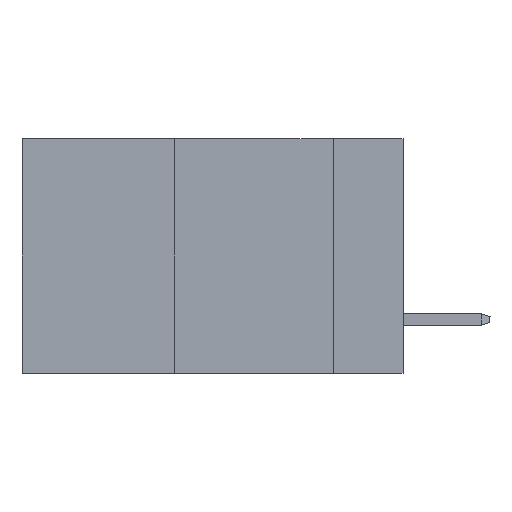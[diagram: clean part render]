
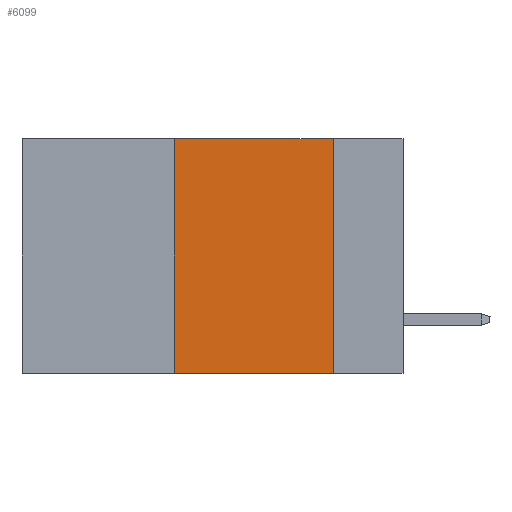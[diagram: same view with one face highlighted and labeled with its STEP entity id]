
A CAD part, left-side view. The second image highlights one B-rep face of the part: STEP entity #6099.
In plain terms, the highlighted planar face has unit normal (-1, 0, 0).
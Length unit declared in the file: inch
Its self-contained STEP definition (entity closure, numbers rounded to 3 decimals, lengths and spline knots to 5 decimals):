
#241 = CARTESIAN_POINT ( 'NONE',  ( 0., 0.36, 0. ) ) ;
#1023 = ORIENTED_EDGE ( 'NONE', *, *, #4505, .F. ) ;
#1237 = DIRECTION ( 'NONE',  ( 0., -1., 0. ) ) ;
#1549 = EDGE_CURVE ( 'NONE', #7417, #3762, #4539, .T. ) ;
#2240 = EDGE_CURVE ( 'NONE', #9723, #2845, #4212, .T. ) ;
#2838 = LINE ( 'NONE', #8310, #6715 ) ;
#2845 = VERTEX_POINT ( 'NONE', #6934 ) ;
#3624 = CARTESIAN_POINT ( 'NONE',  ( 0., 0.11, 0. ) ) ;
#3726 = AXIS2_PLACEMENT_3D ( 'NONE', #7820, #4575, #7723 ) ;
#3762 = VERTEX_POINT ( 'NONE', #6810 ) ;
#4212 = LINE ( 'NONE', #241, #9949 ) ;
#4505 = EDGE_CURVE ( 'NONE', #2845, #7417, #5987, .T. ) ;
#4539 = LINE ( 'NONE', #3624, #6779 ) ;
#4575 = DIRECTION ( 'NONE',  ( 1., 0., 0. ) ) ;
#4925 = EDGE_CURVE ( 'NONE', #9723, #3762, #2838, .T. ) ;
#5872 = CARTESIAN_POINT ( 'NONE',  ( 0., 0.36, -0.37 ) ) ;
#5964 = EDGE_LOOP ( 'NONE', ( #7083, #1023, #9057, #7459 ) ) ;
#5987 = LINE ( 'NONE', #8374, #10152 ) ;
#6099 = ADVANCED_FACE ( 'NONE', ( #10129 ), #6839, .F. ) ;
#6154 = CARTESIAN_POINT ( 'NONE',  ( 0., 0.11, 0. ) ) ;
#6680 = DIRECTION ( 'NONE',  ( 0., 0., -1. ) ) ;
#6715 = VECTOR ( 'NONE', #1237, 39.37008 ) ;
#6779 = VECTOR ( 'NONE', #6680, 39.37008 ) ;
#6810 = CARTESIAN_POINT ( 'NONE',  ( 0., 0.11, -0.37 ) ) ;
#6839 = PLANE ( 'NONE',  #3726 ) ;
#6934 = CARTESIAN_POINT ( 'NONE',  ( 0., 0.36, 0. ) ) ;
#7083 = ORIENTED_EDGE ( 'NONE', *, *, #1549, .F. ) ;
#7417 = VERTEX_POINT ( 'NONE', #6154 ) ;
#7459 = ORIENTED_EDGE ( 'NONE', *, *, #4925, .T. ) ;
#7723 = DIRECTION ( 'NONE',  ( 0., 0., -1. ) ) ;
#7820 = CARTESIAN_POINT ( 'NONE',  ( 0., 0.6, 0. ) ) ;
#8147 = DIRECTION ( 'NONE',  ( 0., 0., 1. ) ) ;
#8310 = CARTESIAN_POINT ( 'NONE',  ( 0., 0.6, -0.37 ) ) ;
#8374 = CARTESIAN_POINT ( 'NONE',  ( 0., 0.6, 0. ) ) ;
#9057 = ORIENTED_EDGE ( 'NONE', *, *, #2240, .F. ) ;
#9148 = DIRECTION ( 'NONE',  ( 0., -1., 0. ) ) ;
#9723 = VERTEX_POINT ( 'NONE', #5872 ) ;
#9949 = VECTOR ( 'NONE', #8147, 39.37008 ) ;
#10129 = FACE_OUTER_BOUND ( 'NONE', #5964, .T. ) ;
#10152 = VECTOR ( 'NONE', #9148, 39.37008 ) ;
